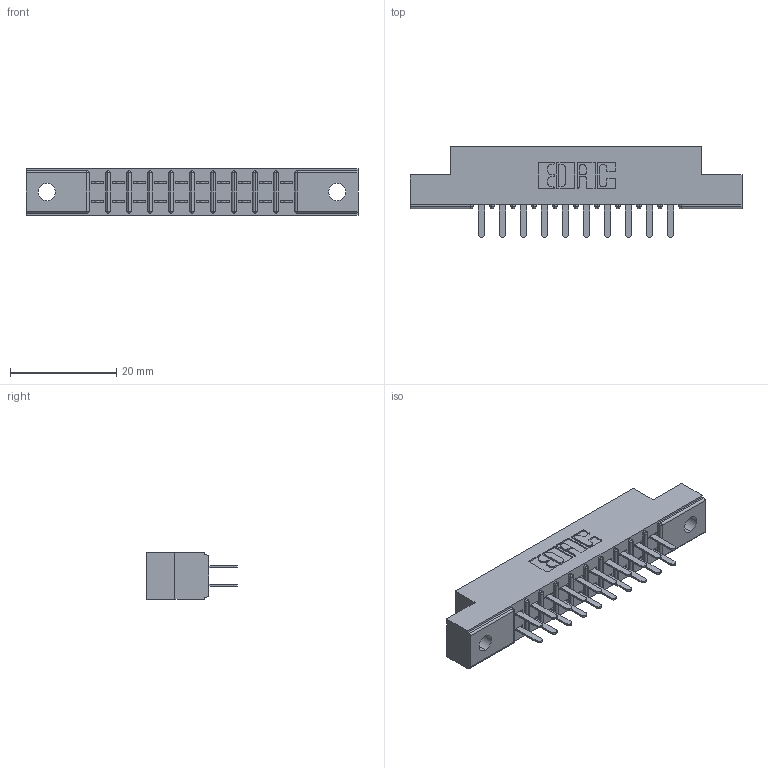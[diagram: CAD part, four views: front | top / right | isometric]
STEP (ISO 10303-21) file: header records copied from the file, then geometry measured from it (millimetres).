
FILE_DESCRIPTION (( 'STEP AP203' ), '1' );
FILE_NAME ('315-020-520-202.STEP', '2019-09-10T14:10:33', ( '' ), ( '' ), 'SwSTEP 2.0', 'SolidWorks 2016', '' );
FILE_SCHEMA (( 'CONFIG_CONTROL_DESIGN' ));
Length unit declared in the file: inch
Products named in the file (3): 305-290-001_520; 315-020-520-202; 305 Part_.128 Dia
Assembly tree (21 placements, depth 2):
  315-020-520-202
    305 Part_.128 Dia
    305-290-001_520  x20
Bounding box: 62.64 x 17.09 x 8.71 mm (x, y, z)
Volume: 3912.3 mm3; surface area: 6435.4 mm2
Topology: 21 solids, 21 shells, 1036 faces, 2946 edges, 1908 vertices
Faces by surface type: plane 608, cylinder 388, sphere 40
Entity records: 14605 total; most frequent: CARTESIAN_POINT 2416, ORIENTED_EDGE 2392, DIRECTION 2362, EDGE_CURVE 1196, LINE 934, VECTOR 934, VERTEX_POINT 768, AXIS2_PLACEMENT_3D 714
